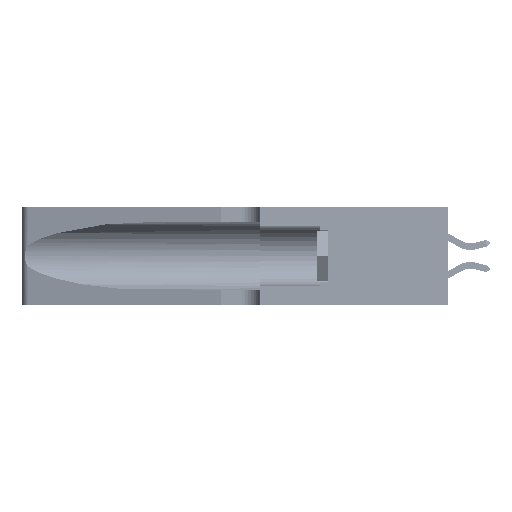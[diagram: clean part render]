
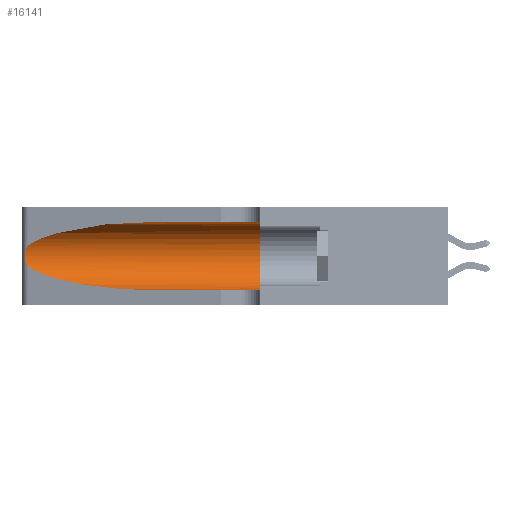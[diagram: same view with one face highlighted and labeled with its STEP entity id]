
A CAD part, left-side view. The second image highlights one B-rep face of the part: STEP entity #16141.
In plain terms, the highlighted cylindrical face has radius 3.308 mm (diameter 6.617 mm), a partial arc.
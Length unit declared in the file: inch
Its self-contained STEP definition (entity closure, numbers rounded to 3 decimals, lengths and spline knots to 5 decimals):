
#1368 = AXIS2_PLACEMENT_3D ( 'NONE', #2926, #42953, #27165 ) ;
#2926 = CARTESIAN_POINT ( 'NONE',  ( 0.1305, 0.35, 0.185 ) ) ;
#4141 = CARTESIAN_POINT ( 'NONE',  ( 0.1305, 0.35, 0.31525 ) ) ;
#4261 = B_SPLINE_CURVE_WITH_KNOTS ( 'NONE', 3,
 ( #43503, #19190, #15132, #35389, #27029, #27206, #43671, #19520, #47523, #23570, #27551, #19702, #47688, #6944 ),
 .UNSPECIFIED., .F., .F.,
 ( 4, 2, 2, 2, 2, 2, 4 ),
 ( 0., 0.00027, 0.00053, 0.00107, 0.0016, 0.00187, 0.00214 ),
 .UNSPECIFIED. ) ;
#5518 = ORIENTED_EDGE ( 'NONE', *, *, #45620, .T. ) ;
#5572 = CARTESIAN_POINT ( 'NONE',  ( 0.18966, 0.96281, 0.31525 ) ) ;
#5972 = VERTEX_POINT ( 'NONE', #4141 ) ;
#6542 = CARTESIAN_POINT ( 'NONE',  ( 0.2373, 1.15595, 0.08982 ) ) ;
#6769 = VECTOR ( 'NONE', #11412, 39.37008 ) ;
#6944 = CARTESIAN_POINT ( 'NONE',  ( 0.25487, 1.22718, 0.14631 ) ) ;
#8471 = CARTESIAN_POINT ( 'NONE',  ( 0.25487, 1.22718, 0.14631 ) ) ;
#8494 = CIRCLE ( 'NONE', #1368, 0.13025 ) ;
#11412 = DIRECTION ( 'NONE',  ( 0., -1., 0. ) ) ;
#11526 = CARTESIAN_POINT ( 'NONE',  ( 0.1305, 0.72297, 0.31525 ) ) ;
#11771 = CARTESIAN_POINT ( 'NONE',  ( 0.1305, 1.61858, 0.05475 ) ) ;
#12204 = ORIENTED_EDGE ( 'NONE', *, *, #50882, .T. ) ;
#12515 = ORIENTED_EDGE ( 'NONE', *, *, #43286, .F. ) ;
#12879 = VERTEX_POINT ( 'NONE', #44385 ) ;
#13080 = CARTESIAN_POINT ( 'NONE',  ( 0.25487, 1.22718, 0.22369 ) ) ;
#15132 = CARTESIAN_POINT ( 'NONE',  ( 0.25639, 1.23184, 0.21858 ) ) ;
#15355 = EDGE_LOOP ( 'NONE', ( #42751, #5518, #19056, #12204, #47364, #12515 ) ) ;
#16141 = ADVANCED_FACE ( 'NONE', ( #50867 ), #38302, .F. ) ;
#16381 = AXIS2_PLACEMENT_3D ( 'NONE', #38749, #23399, #42807 ) ;
#17952 = CARTESIAN_POINT ( 'NONE',  ( 0.1305, 1.61858, 0.31525 ) ) ;
#18691 = EDGE_CURVE ( 'NONE', #20349, #12879, #38838, .T. ) ;
#19056 = ORIENTED_EDGE ( 'NONE', *, *, #24682, .T. ) ;
#19190 = CARTESIAN_POINT ( 'NONE',  ( 0.25555, 1.22994, 0.2215 ) ) ;
#19520 = CARTESIAN_POINT ( 'NONE',  ( 0.26075, 1.23896, 0.178 ) ) ;
#19702 = CARTESIAN_POINT ( 'NONE',  ( 0.25639, 1.23186, 0.15144 ) ) ;
#20349 = VERTEX_POINT ( 'NONE', #11526 ) ;
#20958 = CARTESIAN_POINT ( 'NONE',  ( 0.2373, 1.15595, 0.28018 ) ) ;
#22277 = CARTESIAN_POINT ( 'NONE',  ( 0.1305, 0.72297, 0.05475 ) ) ;
#22633 = CARTESIAN_POINT ( 'NONE',  ( 0.25487, 1.22718, 0.14631 ) ) ;
#23399 = DIRECTION ( 'NONE',  ( 0., -1., 0. ) ) ;
#23570 = CARTESIAN_POINT ( 'NONE',  ( 0.25856, 1.23593, 0.16098 ) ) ;
#24682 = EDGE_CURVE ( 'NONE', #25196, #35081, #32448, .T. ) ;
#25195 = CARTESIAN_POINT ( 'NONE',  ( 0.1305, 0.72297, 0.05475 ) ) ;
#25196 = VERTEX_POINT ( 'NONE', #8471 ) ;
#26109 = CARTESIAN_POINT ( 'NONE',  ( 0.18966, 0.96281, 0.05475 ) ) ;
#26153 = DIRECTION ( 'NONE',  ( 0., -1., 0. ) ) ;
#27029 = CARTESIAN_POINT ( 'NONE',  ( 0.25854, 1.2359, 0.20912 ) ) ;
#27165 = DIRECTION ( 'NONE',  ( 0., 0., 1. ) ) ;
#27206 = CARTESIAN_POINT ( 'NONE',  ( 0.26018, 1.23835, 0.19895 ) ) ;
#27551 = CARTESIAN_POINT ( 'NONE',  ( 0.25789, 1.23486, 0.15765 ) ) ;
#28463 = CARTESIAN_POINT ( 'NONE',  ( 0.1305, 0.35, 0.05475 ) ) ;
#32448 =( BOUNDED_CURVE ( )  B_SPLINE_CURVE ( 3, ( #22633, #6542, #26109, #22277 ),
 .UNSPECIFIED., .F., .T. ) 
 B_SPLINE_CURVE_WITH_KNOTS ( ( 4, 4 ),
 ( 3.44316, 4.71239 ),
 .UNSPECIFIED. ) 
 CURVE ( )  GEOMETRIC_REPRESENTATION_ITEM ( )  RATIONAL_B_SPLINE_CURVE ( ( 1., 0.87, 0.87, 1. ) ) 
 REPRESENTATION_ITEM ( '' )  );
#35081 = VERTEX_POINT ( 'NONE', #25195 ) ;
#35389 = CARTESIAN_POINT ( 'NONE',  ( 0.25787, 1.23484, 0.2124 ) ) ;
#38302 = CYLINDRICAL_SURFACE ( 'NONE', #16381, 0.13025 ) ;
#38596 = LINE ( 'NONE', #11771, #6769 ) ;
#38730 = EDGE_CURVE ( 'NONE', #5972, #49509, #8494, .T. ) ;
#38749 = CARTESIAN_POINT ( 'NONE',  ( 0.1305, 1.61858, 0.185 ) ) ;
#38838 =( BOUNDED_CURVE ( )  B_SPLINE_CURVE ( 3, ( #45119, #5572, #20958, #13080 ),
 .UNSPECIFIED., .F., .F. ) 
 B_SPLINE_CURVE_WITH_KNOTS ( ( 4, 4 ),
 ( 1.5708, 2.84003 ),
 .UNSPECIFIED. ) 
 CURVE ( )  GEOMETRIC_REPRESENTATION_ITEM ( )  RATIONAL_B_SPLINE_CURVE ( ( 1., 0.87, 0.87, 1. ) ) 
 REPRESENTATION_ITEM ( '' )  );
#42751 = ORIENTED_EDGE ( 'NONE', *, *, #18691, .T. ) ;
#42807 = DIRECTION ( 'NONE',  ( 0., 0., -1. ) ) ;
#42953 = DIRECTION ( 'NONE',  ( 0., 1., 0. ) ) ;
#43286 = EDGE_CURVE ( 'NONE', #20349, #5972, #48160, .T. ) ;
#43503 = CARTESIAN_POINT ( 'NONE',  ( 0.25487, 1.22718, 0.22369 ) ) ;
#43671 = CARTESIAN_POINT ( 'NONE',  ( 0.26075, 1.23896, 0.19203 ) ) ;
#44385 = CARTESIAN_POINT ( 'NONE',  ( 0.25487, 1.22718, 0.22369 ) ) ;
#45119 = CARTESIAN_POINT ( 'NONE',  ( 0.1305, 0.72297, 0.31525 ) ) ;
#45620 = EDGE_CURVE ( 'NONE', #12879, #25196, #4261, .T. ) ;
#47364 = ORIENTED_EDGE ( 'NONE', *, *, #38730, .F. ) ;
#47481 = VECTOR ( 'NONE', #26153, 39.37008 ) ;
#47523 = CARTESIAN_POINT ( 'NONE',  ( 0.26017, 1.23833, 0.17102 ) ) ;
#47688 = CARTESIAN_POINT ( 'NONE',  ( 0.25555, 1.22993, 0.14849 ) ) ;
#48160 = LINE ( 'NONE', #17952, #47481 ) ;
#49509 = VERTEX_POINT ( 'NONE', #28463 ) ;
#50867 = FACE_OUTER_BOUND ( 'NONE', #15355, .T. ) ;
#50882 = EDGE_CURVE ( 'NONE', #35081, #49509, #38596, .T. ) ;
